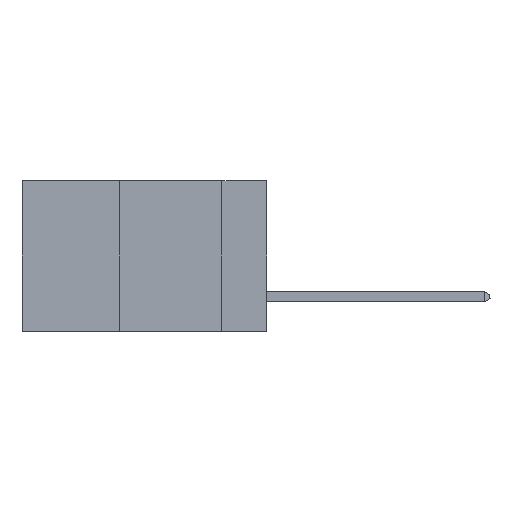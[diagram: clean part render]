
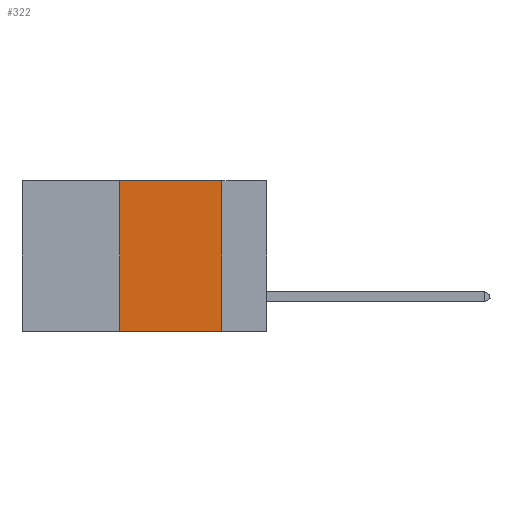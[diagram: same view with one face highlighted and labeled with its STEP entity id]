
A CAD part, left-side view. The second image highlights one B-rep face of the part: STEP entity #322.
In plain terms, the highlighted planar face has unit normal (-1, 0, 0).
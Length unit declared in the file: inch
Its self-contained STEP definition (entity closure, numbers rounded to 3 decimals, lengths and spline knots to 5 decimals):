
#277 = DIRECTION ( 'NONE',  ( 0., 0., -1. ) ) ;
#322 = ADVANCED_FACE ( 'NONE', ( #4844 ), #8389, .F. ) ;
#1915 = AXIS2_PLACEMENT_3D ( 'NONE', #15748, #6465, #13663 ) ;
#2429 = LINE ( 'NONE', #23650, #19627 ) ;
#2739 = EDGE_CURVE ( 'NONE', #20752, #10657, #12461, .T. ) ;
#3712 = CARTESIAN_POINT ( 'NONE',  ( 0., 0.6, -0.37 ) ) ;
#4061 = ORIENTED_EDGE ( 'NONE', *, *, #22495, .F. ) ;
#4844 = FACE_OUTER_BOUND ( 'NONE', #16731, .T. ) ;
#5530 = VECTOR ( 'NONE', #18160, 39.37008 ) ;
#6465 = DIRECTION ( 'NONE',  ( 1., 0., 0. ) ) ;
#7678 = CARTESIAN_POINT ( 'NONE',  ( 0., 0.11, 0. ) ) ;
#8389 = PLANE ( 'NONE',  #1915 ) ;
#8697 = VERTEX_POINT ( 'NONE', #23420 ) ;
#10657 = VERTEX_POINT ( 'NONE', #22948 ) ;
#11389 = EDGE_CURVE ( 'NONE', #16355, #10657, #15546, .T. ) ;
#11938 = ORIENTED_EDGE ( 'NONE', *, *, #21389, .F. ) ;
#12461 = LINE ( 'NONE', #3712, #23705 ) ;
#12731 = DIRECTION ( 'NONE',  ( 0., -1., 0. ) ) ;
#13663 = DIRECTION ( 'NONE',  ( 0., 0., -1. ) ) ;
#15434 = ORIENTED_EDGE ( 'NONE', *, *, #2739, .T. ) ;
#15546 = LINE ( 'NONE', #7678, #21303 ) ;
#15748 = CARTESIAN_POINT ( 'NONE',  ( 0., 0.6, 0. ) ) ;
#15978 = CARTESIAN_POINT ( 'NONE',  ( 0., 0.6, 0. ) ) ;
#16355 = VERTEX_POINT ( 'NONE', #17718 ) ;
#16731 = EDGE_LOOP ( 'NONE', ( #23180, #11938, #4061, #15434 ) ) ;
#17603 = LINE ( 'NONE', #15978, #5530 ) ;
#17718 = CARTESIAN_POINT ( 'NONE',  ( 0., 0.11, 0. ) ) ;
#18160 = DIRECTION ( 'NONE',  ( 0., -1., 0. ) ) ;
#19627 = VECTOR ( 'NONE', #20620, 39.37008 ) ;
#20620 = DIRECTION ( 'NONE',  ( 0., 0., 1. ) ) ;
#20752 = VERTEX_POINT ( 'NONE', #23496 ) ;
#21303 = VECTOR ( 'NONE', #277, 39.37008 ) ;
#21389 = EDGE_CURVE ( 'NONE', #8697, #16355, #17603, .T. ) ;
#22495 = EDGE_CURVE ( 'NONE', #20752, #8697, #2429, .T. ) ;
#22948 = CARTESIAN_POINT ( 'NONE',  ( 0., 0.11, -0.37 ) ) ;
#23180 = ORIENTED_EDGE ( 'NONE', *, *, #11389, .F. ) ;
#23420 = CARTESIAN_POINT ( 'NONE',  ( 0., 0.36, 0. ) ) ;
#23496 = CARTESIAN_POINT ( 'NONE',  ( 0., 0.36, -0.37 ) ) ;
#23650 = CARTESIAN_POINT ( 'NONE',  ( 0., 0.36, 0. ) ) ;
#23705 = VECTOR ( 'NONE', #12731, 39.37008 ) ;
